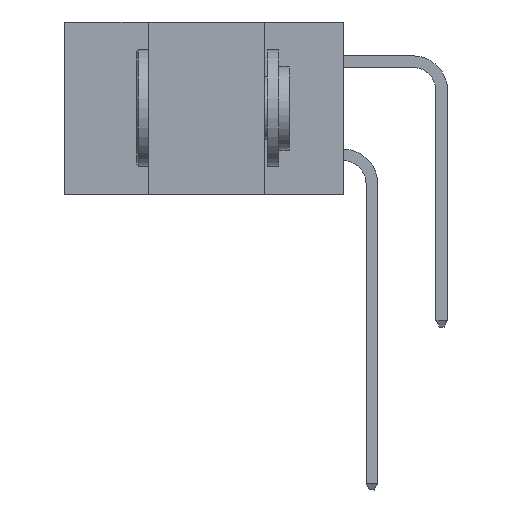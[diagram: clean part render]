
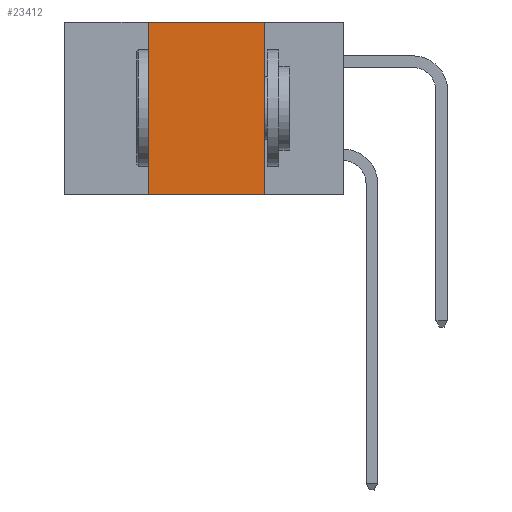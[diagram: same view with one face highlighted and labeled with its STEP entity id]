
A CAD part, left-side view. The second image highlights one B-rep face of the part: STEP entity #23412.
In plain terms, the highlighted planar face has unit normal (-1, 0, 0).
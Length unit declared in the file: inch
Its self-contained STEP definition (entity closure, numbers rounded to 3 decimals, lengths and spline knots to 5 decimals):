
#714 = FACE_OUTER_BOUND ( 'NONE', #4775, .T. ) ;
#922 = ORIENTED_EDGE ( 'NONE', *, *, #10849, .F. ) ;
#993 = VECTOR ( 'NONE', #16128, 39.37008 ) ;
#1041 = DIRECTION ( 'NONE',  ( 0., 0., 1. ) ) ;
#1533 = CARTESIAN_POINT ( 'NONE',  ( 0., 0.42, -0.37 ) ) ;
#2651 = EDGE_CURVE ( 'NONE', #23777, #7350, #12358, .T. ) ;
#2704 = CARTESIAN_POINT ( 'NONE',  ( 0., 0.6, 0. ) ) ;
#4719 = DIRECTION ( 'NONE',  ( 0., 0., -1. ) ) ;
#4775 = EDGE_LOOP ( 'NONE', ( #9268, #20919, #922, #11643 ) ) ;
#6526 = PLANE ( 'NONE',  #17605 ) ;
#7350 = VERTEX_POINT ( 'NONE', #23002 ) ;
#7422 = CARTESIAN_POINT ( 'NONE',  ( 0., 0.17, -0.37 ) ) ;
#8589 = DIRECTION ( 'NONE',  ( 1., 0., 0. ) ) ;
#8902 = CARTESIAN_POINT ( 'NONE',  ( 0., 0.42, -0.37 ) ) ;
#9268 = ORIENTED_EDGE ( 'NONE', *, *, #14027, .F. ) ;
#10720 = VECTOR ( 'NONE', #1041, 39.37008 ) ;
#10849 = EDGE_CURVE ( 'NONE', #13696, #23777, #16670, .T. ) ;
#11263 = CARTESIAN_POINT ( 'NONE',  ( 0., 0.6, -0.37 ) ) ;
#11643 = ORIENTED_EDGE ( 'NONE', *, *, #15837, .T. ) ;
#12358 = LINE ( 'NONE', #2704, #993 ) ;
#13593 = LINE ( 'NONE', #7422, #16979 ) ;
#13696 = VERTEX_POINT ( 'NONE', #1533 ) ;
#14027 = EDGE_CURVE ( 'NONE', #7350, #23338, #13593, .T. ) ;
#15837 = EDGE_CURVE ( 'NONE', #13696, #23338, #25351, .T. ) ;
#16128 = DIRECTION ( 'NONE',  ( 0., -1., 0. ) ) ;
#16202 = VECTOR ( 'NONE', #19268, 39.37008 ) ;
#16670 = LINE ( 'NONE', #8902, #10720 ) ;
#16979 = VECTOR ( 'NONE', #23319, 39.37008 ) ;
#17605 = AXIS2_PLACEMENT_3D ( 'NONE', #22285, #8589, #4719 ) ;
#17987 = CARTESIAN_POINT ( 'NONE',  ( 0., 0.42, 0. ) ) ;
#19268 = DIRECTION ( 'NONE',  ( 0., -1., 0. ) ) ;
#20919 = ORIENTED_EDGE ( 'NONE', *, *, #2651, .F. ) ;
#22285 = CARTESIAN_POINT ( 'NONE',  ( 0., 0.6, 0. ) ) ;
#23002 = CARTESIAN_POINT ( 'NONE',  ( 0., 0.17, 0. ) ) ;
#23319 = DIRECTION ( 'NONE',  ( 0., 0., -1. ) ) ;
#23338 = VERTEX_POINT ( 'NONE', #24474 ) ;
#23412 = ADVANCED_FACE ( 'NONE', ( #714 ), #6526, .F. ) ;
#23777 = VERTEX_POINT ( 'NONE', #17987 ) ;
#24474 = CARTESIAN_POINT ( 'NONE',  ( 0., 0.17, -0.37 ) ) ;
#25351 = LINE ( 'NONE', #11263, #16202 ) ;
